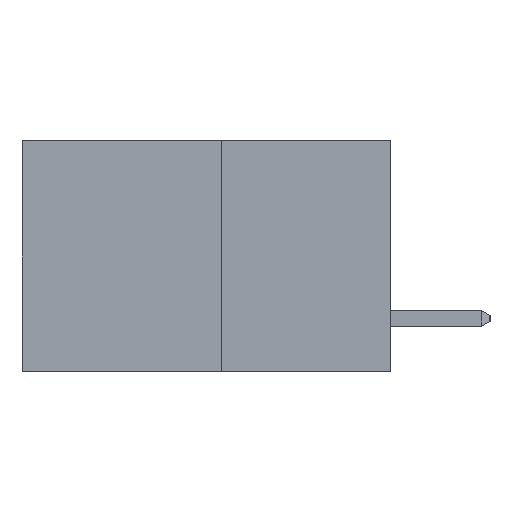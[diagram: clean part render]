
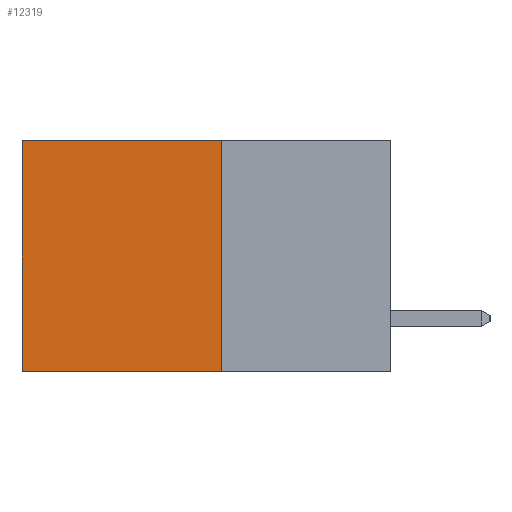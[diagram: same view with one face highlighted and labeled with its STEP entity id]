
A CAD part, left-side view. The second image highlights one B-rep face of the part: STEP entity #12319.
In plain terms, the highlighted planar face has unit normal (-1, 0, 0).
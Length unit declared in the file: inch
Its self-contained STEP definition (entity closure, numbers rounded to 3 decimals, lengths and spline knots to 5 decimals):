
#1066 = VECTOR ( 'NONE', #15257, 39.37008 ) ;
#1287 = VERTEX_POINT ( 'NONE', #4241 ) ;
#2154 = CARTESIAN_POINT ( 'NONE',  ( 0.277, 0.27, 0. ) ) ;
#2335 = CARTESIAN_POINT ( 'NONE',  ( 0.277, 0.27, -0.37 ) ) ;
#3289 = DIRECTION ( 'NONE',  ( 0., 1., 0. ) ) ;
#3672 = EDGE_CURVE ( 'NONE', #22573, #1287, #10931, .T. ) ;
#4180 = DIRECTION ( 'NONE',  ( 0., 1., 0. ) ) ;
#4241 = CARTESIAN_POINT ( 'NONE',  ( 0.277, 0.59, -0.37 ) ) ;
#4500 = PLANE ( 'NONE',  #16488 ) ;
#4545 = CARTESIAN_POINT ( 'NONE',  ( 0.277, 0.27, -0.37 ) ) ;
#5094 = EDGE_CURVE ( 'NONE', #22711, #1287, #20801, .T. ) ;
#6539 = CARTESIAN_POINT ( 'NONE',  ( 0.277, 0.59, 0. ) ) ;
#6780 = VECTOR ( 'NONE', #4180, 39.37008 ) ;
#6948 = CARTESIAN_POINT ( 'NONE',  ( 0.277, 0.27, -0.37 ) ) ;
#8163 = DIRECTION ( 'NONE',  ( 0., 0., -1. ) ) ;
#8822 = VECTOR ( 'NONE', #3289, 39.37008 ) ;
#8878 = ORIENTED_EDGE ( 'NONE', *, *, #9586, .T. ) ;
#9317 = ORIENTED_EDGE ( 'NONE', *, *, #3672, .T. ) ;
#9451 = FACE_OUTER_BOUND ( 'NONE', #16667, .T. ) ;
#9586 = EDGE_CURVE ( 'NONE', #14033, #22573, #22775, .T. ) ;
#10373 = VECTOR ( 'NONE', #12270, 39.37008 ) ;
#10931 = LINE ( 'NONE', #12524, #10373 ) ;
#12270 = DIRECTION ( 'NONE',  ( 0., 0., -1. ) ) ;
#12319 = ADVANCED_FACE ( 'NONE', ( #9451 ), #4500, .F. ) ;
#12524 = CARTESIAN_POINT ( 'NONE',  ( 0.277, 0.59, -0.37 ) ) ;
#14033 = VERTEX_POINT ( 'NONE', #2154 ) ;
#14097 = ORIENTED_EDGE ( 'NONE', *, *, #5094, .F. ) ;
#15257 = DIRECTION ( 'NONE',  ( 0., 0., -1. ) ) ;
#15343 = LINE ( 'NONE', #4545, #1066 ) ;
#16488 = AXIS2_PLACEMENT_3D ( 'NONE', #16939, #18671, #8163 ) ;
#16568 = EDGE_CURVE ( 'NONE', #14033, #22711, #15343, .T. ) ;
#16667 = EDGE_LOOP ( 'NONE', ( #9317, #14097, #20865, #8878 ) ) ;
#16939 = CARTESIAN_POINT ( 'NONE',  ( 0.277, 0.27, -0.37 ) ) ;
#17448 = CARTESIAN_POINT ( 'NONE',  ( 0.277, 0.27, 0. ) ) ;
#18671 = DIRECTION ( 'NONE',  ( 1., 0., 0. ) ) ;
#20801 = LINE ( 'NONE', #2335, #6780 ) ;
#20865 = ORIENTED_EDGE ( 'NONE', *, *, #16568, .F. ) ;
#22573 = VERTEX_POINT ( 'NONE', #6539 ) ;
#22711 = VERTEX_POINT ( 'NONE', #6948 ) ;
#22775 = LINE ( 'NONE', #17448, #8822 ) ;
